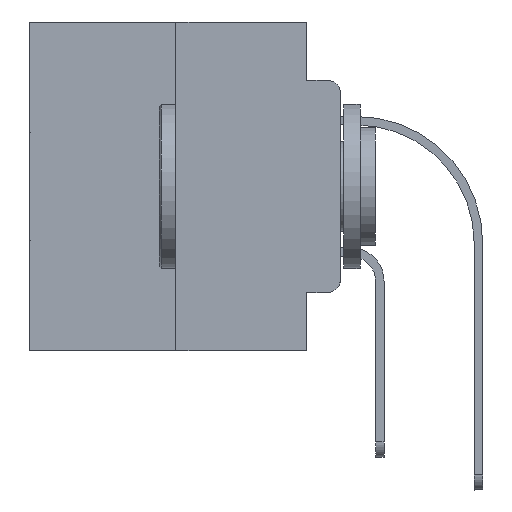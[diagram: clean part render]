
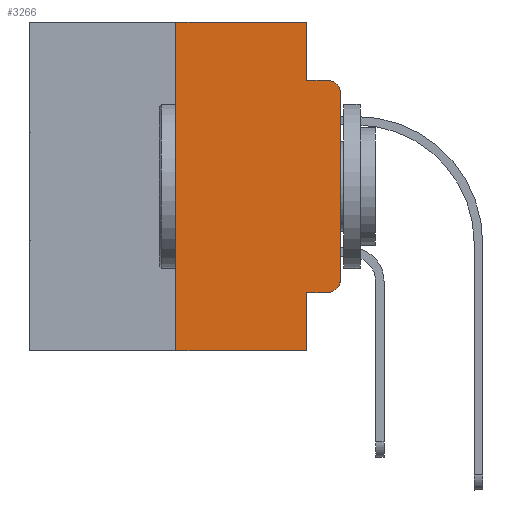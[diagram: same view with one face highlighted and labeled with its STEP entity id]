
A CAD part, left-side view. The second image highlights one B-rep face of the part: STEP entity #3266.
In plain terms, the highlighted planar face has unit normal (-1, 0, 0).
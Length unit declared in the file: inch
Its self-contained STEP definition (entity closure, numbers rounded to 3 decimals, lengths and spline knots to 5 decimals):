
#210 = CARTESIAN_POINT ( 'NONE',  ( 0., 0., -0.3915 ) ) ;
#610 = VERTEX_POINT ( 'NONE', #30321 ) ;
#2132 = CARTESIAN_POINT ( 'NONE',  ( 0., 0.02, -0.3915 ) ) ;
#2166 = DIRECTION ( 'NONE',  ( 0., 0., -1. ) ) ;
#2167 = VECTOR ( 'NONE', #19066, 39.37008 ) ;
#2636 = LINE ( 'NONE', #7543, #11101 ) ;
#3243 = VERTEX_POINT ( 'NONE', #11359 ) ;
#3266 = ADVANCED_FACE ( 'NONE', ( #25857 ), #8663, .F. ) ;
#3432 = VERTEX_POINT ( 'NONE', #19186 ) ;
#3462 = CARTESIAN_POINT ( 'NONE',  ( 0., 0.051, -0.4115 ) ) ;
#3549 = LINE ( 'NONE', #13248, #29479 ) ;
#4026 = LINE ( 'NONE', #13729, #21420 ) ;
#4890 = DIRECTION ( 'NONE',  ( -1., 0., 0. ) ) ;
#5160 = AXIS2_PLACEMENT_3D ( 'NONE', #2132, #16773, #6892 ) ;
#5602 = ORIENTED_EDGE ( 'NONE', *, *, #12893, .F. ) ;
#5675 = CARTESIAN_POINT ( 'NONE',  ( 0., 0.051, 0. ) ) ;
#6892 = DIRECTION ( 'NONE',  ( 0., 0., -1. ) ) ;
#7543 = CARTESIAN_POINT ( 'NONE',  ( 0., 0.051, 0. ) ) ;
#8663 = PLANE ( 'NONE',  #19863 ) ;
#8687 = LINE ( 'NONE', #5675, #26419 ) ;
#9355 = VERTEX_POINT ( 'NONE', #24401 ) ;
#9752 = CARTESIAN_POINT ( 'NONE',  ( 0., 0.473, -0.5 ) ) ;
#10049 = EDGE_CURVE ( 'NONE', #24633, #610, #17620, .T. ) ;
#10058 = ORIENTED_EDGE ( 'NONE', *, *, #28095, .F. ) ;
#10347 = EDGE_CURVE ( 'NONE', #23349, #21711, #21698, .T. ) ;
#10598 = ORIENTED_EDGE ( 'NONE', *, *, #28036, .T. ) ;
#10625 = ORIENTED_EDGE ( 'NONE', *, *, #30341, .T. ) ;
#10980 = CARTESIAN_POINT ( 'NONE',  ( 0., 0., -0.1085 ) ) ;
#11101 = VECTOR ( 'NONE', #2166, 39.37008 ) ;
#11268 = VERTEX_POINT ( 'NONE', #19235 ) ;
#11359 = CARTESIAN_POINT ( 'NONE',  ( 0., 0.051, 0. ) ) ;
#11538 = VECTOR ( 'NONE', #16775, 39.37008 ) ;
#11819 = DIRECTION ( 'NONE',  ( 0., -1., 0. ) ) ;
#11826 = EDGE_CURVE ( 'NONE', #3243, #9355, #2636, .T. ) ;
#12893 = EDGE_CURVE ( 'NONE', #3432, #21711, #8687, .T. ) ;
#13248 = CARTESIAN_POINT ( 'NONE',  ( 0., 0.25, 0. ) ) ;
#13480 = DIRECTION ( 'NONE',  ( 0., -1., 0. ) ) ;
#13729 = CARTESIAN_POINT ( 'NONE',  ( 0., 0.473, 0. ) ) ;
#13812 = CARTESIAN_POINT ( 'NONE',  ( 0., 0.02, -0.1085 ) ) ;
#13918 = DIRECTION ( 'NONE',  ( 1., 0., 0. ) ) ;
#14049 = CARTESIAN_POINT ( 'NONE',  ( 0., 0.051, -0.5 ) ) ;
#14569 = ORIENTED_EDGE ( 'NONE', *, *, #29002, .T. ) ;
#14603 = DIRECTION ( 'NONE',  ( 0., 0., -1. ) ) ;
#14898 = ORIENTED_EDGE ( 'NONE', *, *, #27603, .F. ) ;
#15416 = ORIENTED_EDGE ( 'NONE', *, *, #10049, .T. ) ;
#16288 = VECTOR ( 'NONE', #13480, 39.37008 ) ;
#16659 = LINE ( 'NONE', #21270, #2167 ) ;
#16673 = CARTESIAN_POINT ( 'NONE',  ( 0., 0.051, -0.0885 ) ) ;
#16773 = DIRECTION ( 'NONE',  ( -1., 0., 0. ) ) ;
#16775 = DIRECTION ( 'NONE',  ( 0., -1., 0. ) ) ;
#17620 = CIRCLE ( 'NONE', #21706, 0.02 ) ;
#17775 = DIRECTION ( 'NONE',  ( 0., 0., -1. ) ) ;
#18531 = ORIENTED_EDGE ( 'NONE', *, *, #10347, .T. ) ;
#19066 = DIRECTION ( 'NONE',  ( 0., 0., 1. ) ) ;
#19186 = CARTESIAN_POINT ( 'NONE',  ( 0., 0.051, -0.4115 ) ) ;
#19235 = CARTESIAN_POINT ( 'NONE',  ( 0., 0.25, 0. ) ) ;
#19401 = CIRCLE ( 'NONE', #5160, 0.02 ) ;
#19636 = EDGE_LOOP ( 'NONE', ( #10625, #15416, #10058, #27570, #30954, #14898, #18531, #5602, #10598, #14569 ) ) ;
#19863 = AXIS2_PLACEMENT_3D ( 'NONE', #23483, #13918, #28746 ) ;
#21270 = CARTESIAN_POINT ( 'NONE',  ( 0., 0., 0. ) ) ;
#21420 = VECTOR ( 'NONE', #11819, 39.37008 ) ;
#21698 = LINE ( 'NONE', #9752, #11538 ) ;
#21706 = AXIS2_PLACEMENT_3D ( 'NONE', #13812, #4890, #14603 ) ;
#21711 = VERTEX_POINT ( 'NONE', #14049 ) ;
#21766 = LINE ( 'NONE', #16673, #27454 ) ;
#23349 = VERTEX_POINT ( 'NONE', #28027 ) ;
#23403 = DIRECTION ( 'NONE',  ( 0., 0., 1. ) ) ;
#23483 = CARTESIAN_POINT ( 'NONE',  ( 0., 0.473, 0. ) ) ;
#24008 = DIRECTION ( 'NONE',  ( 0., -1., 0. ) ) ;
#24401 = CARTESIAN_POINT ( 'NONE',  ( 0., 0.051, -0.0885 ) ) ;
#24633 = VERTEX_POINT ( 'NONE', #10980 ) ;
#25556 = VERTEX_POINT ( 'NONE', #26520 ) ;
#25857 = FACE_OUTER_BOUND ( 'NONE', #19636, .T. ) ;
#26419 = VECTOR ( 'NONE', #17775, 39.37008 ) ;
#26520 = CARTESIAN_POINT ( 'NONE',  ( 0., 0.02, -0.4115 ) ) ;
#27454 = VECTOR ( 'NONE', #24008, 39.37008 ) ;
#27570 = ORIENTED_EDGE ( 'NONE', *, *, #11826, .F. ) ;
#27603 = EDGE_CURVE ( 'NONE', #23349, #11268, #3549, .T. ) ;
#28027 = CARTESIAN_POINT ( 'NONE',  ( 0., 0.25, -0.5 ) ) ;
#28036 = EDGE_CURVE ( 'NONE', #3432, #25556, #30545, .T. ) ;
#28095 = EDGE_CURVE ( 'NONE', #9355, #610, #21766, .T. ) ;
#28746 = DIRECTION ( 'NONE',  ( 0., 0., -1. ) ) ;
#29002 = EDGE_CURVE ( 'NONE', #25556, #29175, #19401, .T. ) ;
#29034 = EDGE_CURVE ( 'NONE', #11268, #3243, #4026, .T. ) ;
#29175 = VERTEX_POINT ( 'NONE', #210 ) ;
#29479 = VECTOR ( 'NONE', #23403, 39.37008 ) ;
#30321 = CARTESIAN_POINT ( 'NONE',  ( 0., 0.02, -0.0885 ) ) ;
#30341 = EDGE_CURVE ( 'NONE', #29175, #24633, #16659, .T. ) ;
#30545 = LINE ( 'NONE', #3462, #16288 ) ;
#30954 = ORIENTED_EDGE ( 'NONE', *, *, #29034, .F. ) ;
